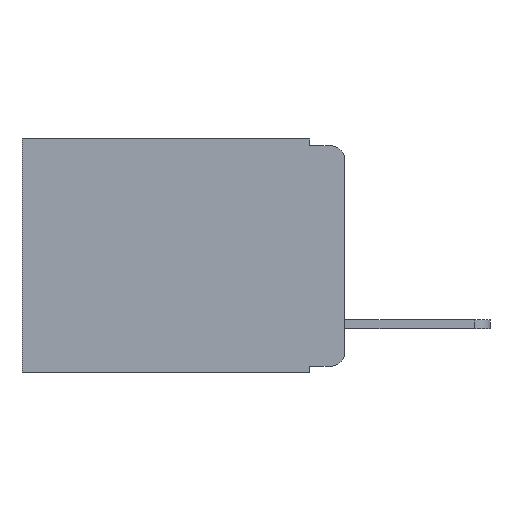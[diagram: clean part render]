
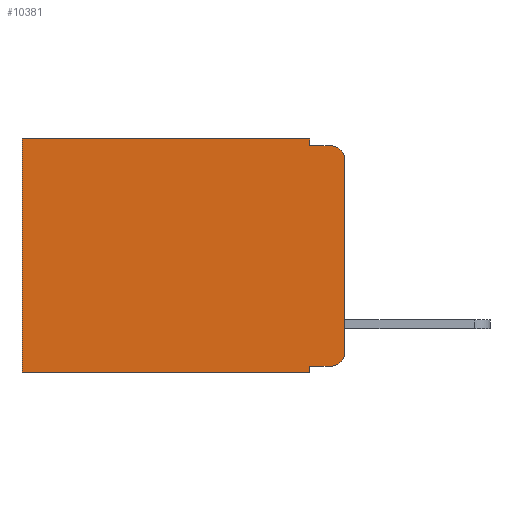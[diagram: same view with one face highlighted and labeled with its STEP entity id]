
A CAD part, left-side view. The second image highlights one B-rep face of the part: STEP entity #10381.
In plain terms, the highlighted planar face has unit normal (-1, 0, 0).
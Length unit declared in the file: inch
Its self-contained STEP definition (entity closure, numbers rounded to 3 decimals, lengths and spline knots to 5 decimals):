
#294 = EDGE_CURVE ( 'NONE', #4249, #4442, #937, .T. ) ;
#695 = DIRECTION ( 'NONE',  ( 0., 0., -1. ) ) ;
#750 = CARTESIAN_POINT ( 'NONE',  ( 0.298, 0.473, 0. ) ) ;
#777 = LINE ( 'NONE', #7393, #3185 ) ;
#937 = CIRCLE ( 'NONE', #1282, 0.02 ) ;
#1027 = CARTESIAN_POINT ( 'NONE',  ( 0.298, 0.473, -0.343 ) ) ;
#1166 = VERTEX_POINT ( 'NONE', #3620 ) ;
#1256 = CARTESIAN_POINT ( 'NONE',  ( 0.298, 0., -0.313 ) ) ;
#1282 = AXIS2_PLACEMENT_3D ( 'NONE', #5686, #8820, #695 ) ;
#1404 = DIRECTION ( 'NONE',  ( 0., 1., 0. ) ) ;
#1665 = VERTEX_POINT ( 'NONE', #750 ) ;
#1720 = VERTEX_POINT ( 'NONE', #2489 ) ;
#1975 = LINE ( 'NONE', #6909, #6703 ) ;
#2057 = EDGE_CURVE ( 'NONE', #1720, #1665, #1975, .T. ) ;
#2489 = CARTESIAN_POINT ( 'NONE',  ( 0.298, 0.051, 0. ) ) ;
#2642 = EDGE_LOOP ( 'NONE', ( #4239, #4131, #9158, #4063, #7237, #4014, #7300, #3937, #8792, #3837 ) ) ;
#2806 = VECTOR ( 'NONE', #3027, 39.37008 ) ;
#3027 = DIRECTION ( 'NONE',  ( 0., 0., -1. ) ) ;
#3065 = DIRECTION ( 'NONE',  ( 0., 0., -1. ) ) ;
#3185 = VECTOR ( 'NONE', #3065, 39.37008 ) ;
#3229 = VECTOR ( 'NONE', #9871, 39.37008 ) ;
#3300 = LINE ( 'NONE', #10571, #3575 ) ;
#3552 = CARTESIAN_POINT ( 'NONE',  ( 0.298, 0.051, -0.333 ) ) ;
#3575 = VECTOR ( 'NONE', #5743, 39.37008 ) ;
#3620 = CARTESIAN_POINT ( 'NONE',  ( 0.298, 0.02, -0.333 ) ) ;
#3769 = CARTESIAN_POINT ( 'NONE',  ( 0.298, 0.051, -0.333 ) ) ;
#3837 = ORIENTED_EDGE ( 'NONE', *, *, #4750, .T. ) ;
#3937 = ORIENTED_EDGE ( 'NONE', *, *, #7016, .F. ) ;
#3972 = CARTESIAN_POINT ( 'NONE',  ( 0.298, 0., 0. ) ) ;
#4014 = ORIENTED_EDGE ( 'NONE', *, *, #7578, .T. ) ;
#4063 = ORIENTED_EDGE ( 'NONE', *, *, #8622, .F. ) ;
#4079 = AXIS2_PLACEMENT_3D ( 'NONE', #3972, #10590, #5765 ) ;
#4131 = ORIENTED_EDGE ( 'NONE', *, *, #294, .T. ) ;
#4203 = VECTOR ( 'NONE', #4543, 39.37008 ) ;
#4239 = ORIENTED_EDGE ( 'NONE', *, *, #5717, .F. ) ;
#4249 = VERTEX_POINT ( 'NONE', #6206 ) ;
#4442 = VERTEX_POINT ( 'NONE', #4956 ) ;
#4451 = LINE ( 'NONE', #6710, #7510 ) ;
#4543 = DIRECTION ( 'NONE',  ( 0., 0., -1. ) ) ;
#4750 = EDGE_CURVE ( 'NONE', #1166, #7513, #7950, .T. ) ;
#4956 = CARTESIAN_POINT ( 'NONE',  ( 0.298, 0.02, -0.01 ) ) ;
#5194 = LINE ( 'NONE', #10204, #2806 ) ;
#5608 = LINE ( 'NONE', #10550, #3229 ) ;
#5617 = VECTOR ( 'NONE', #6819, 39.37008 ) ;
#5686 = CARTESIAN_POINT ( 'NONE',  ( 0.298, 0.02, -0.03 ) ) ;
#5717 = EDGE_CURVE ( 'NONE', #4249, #7513, #5194, .T. ) ;
#5743 = DIRECTION ( 'NONE',  ( 0., -1., 0. ) ) ;
#5765 = DIRECTION ( 'NONE',  ( 0., 0., -1. ) ) ;
#5792 = CARTESIAN_POINT ( 'NONE',  ( 0.298, 0.051, -0.343 ) ) ;
#5918 = EDGE_CURVE ( 'NONE', #10081, #1166, #7811, .T. ) ;
#5952 = AXIS2_PLACEMENT_3D ( 'NONE', #10229, #8714, #8677 ) ;
#6206 = CARTESIAN_POINT ( 'NONE',  ( 0.298, 0., -0.03 ) ) ;
#6256 = VERTEX_POINT ( 'NONE', #5792 ) ;
#6516 = LINE ( 'NONE', #9291, #4203 ) ;
#6703 = VECTOR ( 'NONE', #6839, 39.37008 ) ;
#6710 = CARTESIAN_POINT ( 'NONE',  ( 0.298, 0., -0.343 ) ) ;
#6819 = DIRECTION ( 'NONE',  ( 0., -1., 0. ) ) ;
#6839 = DIRECTION ( 'NONE',  ( 0., 1., 0. ) ) ;
#6909 = CARTESIAN_POINT ( 'NONE',  ( 0.298, 0., 0. ) ) ;
#7016 = EDGE_CURVE ( 'NONE', #10081, #6256, #5608, .T. ) ;
#7237 = ORIENTED_EDGE ( 'NONE', *, *, #2057, .T. ) ;
#7300 = ORIENTED_EDGE ( 'NONE', *, *, #8717, .F. ) ;
#7393 = CARTESIAN_POINT ( 'NONE',  ( 0.298, 0.051, 0. ) ) ;
#7510 = VECTOR ( 'NONE', #1404, 39.37008 ) ;
#7513 = VERTEX_POINT ( 'NONE', #1256 ) ;
#7578 = EDGE_CURVE ( 'NONE', #1665, #8455, #6516, .T. ) ;
#7811 = LINE ( 'NONE', #3769, #5617 ) ;
#7950 = CIRCLE ( 'NONE', #5952, 0.02 ) ;
#8241 = FACE_OUTER_BOUND ( 'NONE', #2642, .T. ) ;
#8387 = CARTESIAN_POINT ( 'NONE',  ( 0.298, 0.051, -0.01 ) ) ;
#8455 = VERTEX_POINT ( 'NONE', #1027 ) ;
#8622 = EDGE_CURVE ( 'NONE', #1720, #10527, #777, .T. ) ;
#8677 = DIRECTION ( 'NONE',  ( 0., 0., -1. ) ) ;
#8714 = DIRECTION ( 'NONE',  ( -1., 0., 0. ) ) ;
#8717 = EDGE_CURVE ( 'NONE', #6256, #8455, #4451, .T. ) ;
#8792 = ORIENTED_EDGE ( 'NONE', *, *, #5918, .T. ) ;
#8820 = DIRECTION ( 'NONE',  ( -1., 0., 0. ) ) ;
#8986 = PLANE ( 'NONE',  #4079 ) ;
#9158 = ORIENTED_EDGE ( 'NONE', *, *, #9686, .F. ) ;
#9291 = CARTESIAN_POINT ( 'NONE',  ( 0.298, 0.473, 0. ) ) ;
#9686 = EDGE_CURVE ( 'NONE', #10527, #4442, #3300, .T. ) ;
#9871 = DIRECTION ( 'NONE',  ( 0., 0., -1. ) ) ;
#10081 = VERTEX_POINT ( 'NONE', #3552 ) ;
#10204 = CARTESIAN_POINT ( 'NONE',  ( 0.298, 0., 0. ) ) ;
#10229 = CARTESIAN_POINT ( 'NONE',  ( 0.298, 0.02, -0.313 ) ) ;
#10381 = ADVANCED_FACE ( 'NONE', ( #8241 ), #8986, .F. ) ;
#10527 = VERTEX_POINT ( 'NONE', #8387 ) ;
#10550 = CARTESIAN_POINT ( 'NONE',  ( 0.298, 0.051, 0. ) ) ;
#10571 = CARTESIAN_POINT ( 'NONE',  ( 0.298, 0.051, -0.01 ) ) ;
#10590 = DIRECTION ( 'NONE',  ( 1., 0., 0. ) ) ;
